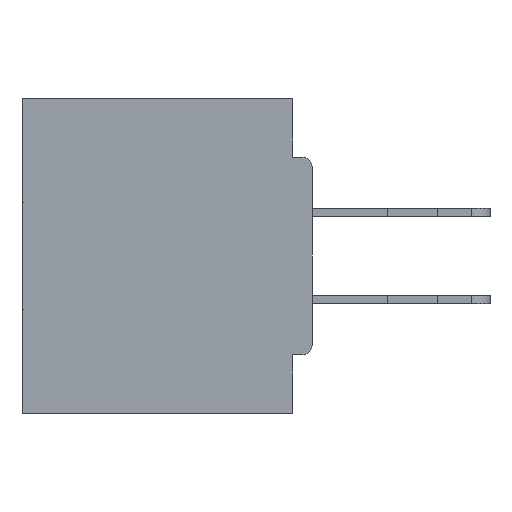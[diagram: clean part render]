
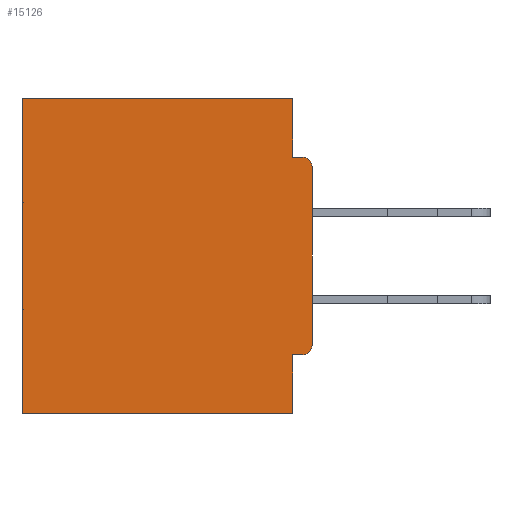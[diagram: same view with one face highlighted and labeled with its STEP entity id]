
A CAD part, left-side view. The second image highlights one B-rep face of the part: STEP entity #15126.
In plain terms, the highlighted planar face has unit normal (-1, 0, 0).
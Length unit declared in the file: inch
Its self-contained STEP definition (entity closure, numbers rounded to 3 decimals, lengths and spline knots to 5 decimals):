
#504 = LINE ( 'NONE', #10023, #5529 ) ;
#1073 = CARTESIAN_POINT ( 'NONE',  ( 0.298, 0.015, -0.4065 ) ) ;
#1632 = EDGE_LOOP ( 'NONE', ( #32074, #9726, #23702, #25996, #10552, #6517, #4201, #10667, #2565, #26177 ) ) ;
#1644 = EDGE_CURVE ( 'NONE', #39556, #12354, #32838, .T. ) ;
#1906 = CARTESIAN_POINT ( 'NONE',  ( 0.298, 0.031, -0.4065 ) ) ;
#2469 = FACE_OUTER_BOUND ( 'NONE', #1632, .T. ) ;
#2565 = ORIENTED_EDGE ( 'NONE', *, *, #34177, .T. ) ;
#2926 = LINE ( 'NONE', #29015, #8430 ) ;
#3971 = EDGE_CURVE ( 'NONE', #5080, #12354, #32629, .T. ) ;
#4201 = ORIENTED_EDGE ( 'NONE', *, *, #24103, .F. ) ;
#5080 = VERTEX_POINT ( 'NONE', #30779 ) ;
#5529 = VECTOR ( 'NONE', #22560, 39.37008 ) ;
#5671 = DIRECTION ( 'NONE',  ( 0., 0., -1. ) ) ;
#6390 = DIRECTION ( 'NONE',  ( 0., 0., -1. ) ) ;
#6517 = ORIENTED_EDGE ( 'NONE', *, *, #10736, .F. ) ;
#7818 = CARTESIAN_POINT ( 'NONE',  ( 0.298, 0., 0. ) ) ;
#8029 = EDGE_CURVE ( 'NONE', #39330, #17224, #26797, .T. ) ;
#8430 = VECTOR ( 'NONE', #19400, 39.37008 ) ;
#8627 = AXIS2_PLACEMENT_3D ( 'NONE', #16144, #38424, #19344 ) ;
#8800 = LINE ( 'NONE', #11497, #19780 ) ;
#9360 = CARTESIAN_POINT ( 'NONE',  ( 0.298, 0.015, -0.1085 ) ) ;
#9726 = ORIENTED_EDGE ( 'NONE', *, *, #1644, .F. ) ;
#10023 = CARTESIAN_POINT ( 'NONE',  ( 0.298, 0., 0. ) ) ;
#10038 = CIRCLE ( 'NONE', #8627, 0.015 ) ;
#10053 = VECTOR ( 'NONE', #5671, 39.37008 ) ;
#10339 = LINE ( 'NONE', #15567, #19294 ) ;
#10552 = ORIENTED_EDGE ( 'NONE', *, *, #19890, .T. ) ;
#10667 = ORIENTED_EDGE ( 'NONE', *, *, #20920, .F. ) ;
#10736 = EDGE_CURVE ( 'NONE', #15590, #25500, #8800, .T. ) ;
#11012 = LINE ( 'NONE', #41060, #10053 ) ;
#11497 = CARTESIAN_POINT ( 'NONE',  ( 0.298, 0., -0.5 ) ) ;
#12354 = VERTEX_POINT ( 'NONE', #16309 ) ;
#12624 = VERTEX_POINT ( 'NONE', #1073 ) ;
#13144 = DIRECTION ( 'NONE',  ( 0., -1., 0. ) ) ;
#13216 = VECTOR ( 'NONE', #37300, 39.37008 ) ;
#14861 = VECTOR ( 'NONE', #13144, 39.37008 ) ;
#15126 = ADVANCED_FACE ( 'NONE', ( #2469 ), #41079, .F. ) ;
#15567 = CARTESIAN_POINT ( 'NONE',  ( 0.298, 0., -0.4065 ) ) ;
#15590 = VERTEX_POINT ( 'NONE', #34446 ) ;
#15785 = CARTESIAN_POINT ( 'NONE',  ( 0.298, 0.031, 0. ) ) ;
#16144 = CARTESIAN_POINT ( 'NONE',  ( 0.298, 0.015, -0.3915 ) ) ;
#16309 = CARTESIAN_POINT ( 'NONE',  ( 0.298, 0.015, -0.0935 ) ) ;
#17224 = VERTEX_POINT ( 'NONE', #37334 ) ;
#18289 = VECTOR ( 'NONE', #39715, 39.37008 ) ;
#18800 = EDGE_CURVE ( 'NONE', #5080, #19635, #504, .T. ) ;
#18860 = CARTESIAN_POINT ( 'NONE',  ( 0.298, 0.46, -0.5 ) ) ;
#18916 = DIRECTION ( 'NONE',  ( 0., 1., 0. ) ) ;
#19294 = VECTOR ( 'NONE', #18916, 39.37008 ) ;
#19344 = DIRECTION ( 'NONE',  ( 0., 0., -1. ) ) ;
#19400 = DIRECTION ( 'NONE',  ( 0., 0., -1. ) ) ;
#19635 = VERTEX_POINT ( 'NONE', #39042 ) ;
#19780 = VECTOR ( 'NONE', #21122, 39.37008 ) ;
#19890 = EDGE_CURVE ( 'NONE', #17224, #25500, #2926, .T. ) ;
#20398 = CARTESIAN_POINT ( 'NONE',  ( 0.298, 0.031, -0.0935 ) ) ;
#20920 = EDGE_CURVE ( 'NONE', #12624, #30329, #10339, .T. ) ;
#21122 = DIRECTION ( 'NONE',  ( 0., 1., 0. ) ) ;
#22560 = DIRECTION ( 'NONE',  ( 0., 0., -1. ) ) ;
#23702 = ORIENTED_EDGE ( 'NONE', *, *, #26275, .F. ) ;
#24103 = EDGE_CURVE ( 'NONE', #30329, #15590, #30160, .T. ) ;
#25359 = DIRECTION ( 'NONE',  ( -1., 0., 0. ) ) ;
#25500 = VERTEX_POINT ( 'NONE', #18860 ) ;
#25996 = ORIENTED_EDGE ( 'NONE', *, *, #8029, .T. ) ;
#26177 = ORIENTED_EDGE ( 'NONE', *, *, #18800, .F. ) ;
#26275 = EDGE_CURVE ( 'NONE', #39330, #39556, #11012, .T. ) ;
#26797 = LINE ( 'NONE', #7818, #18289 ) ;
#28815 = DIRECTION ( 'NONE',  ( 1., 0., 0. ) ) ;
#29015 = CARTESIAN_POINT ( 'NONE',  ( 0.298, 0.46, 0. ) ) ;
#29329 = CARTESIAN_POINT ( 'NONE',  ( 0.298, 0., -0.0935 ) ) ;
#30160 = LINE ( 'NONE', #39994, #13216 ) ;
#30329 = VERTEX_POINT ( 'NONE', #1906 ) ;
#30779 = CARTESIAN_POINT ( 'NONE',  ( 0.298, 0., -0.1085 ) ) ;
#31103 = DIRECTION ( 'NONE',  ( 0., 0., -1. ) ) ;
#31507 = AXIS2_PLACEMENT_3D ( 'NONE', #34912, #28815, #6390 ) ;
#31741 = AXIS2_PLACEMENT_3D ( 'NONE', #9360, #25359, #31103 ) ;
#32074 = ORIENTED_EDGE ( 'NONE', *, *, #3971, .T. ) ;
#32629 = CIRCLE ( 'NONE', #31741, 0.015 ) ;
#32838 = LINE ( 'NONE', #29329, #14861 ) ;
#34177 = EDGE_CURVE ( 'NONE', #12624, #19635, #10038, .T. ) ;
#34446 = CARTESIAN_POINT ( 'NONE',  ( 0.298, 0.031, -0.5 ) ) ;
#34912 = CARTESIAN_POINT ( 'NONE',  ( 0.298, 0., 0. ) ) ;
#37300 = DIRECTION ( 'NONE',  ( 0., 0., -1. ) ) ;
#37334 = CARTESIAN_POINT ( 'NONE',  ( 0.298, 0.46, 0. ) ) ;
#38424 = DIRECTION ( 'NONE',  ( -1., 0., 0. ) ) ;
#39042 = CARTESIAN_POINT ( 'NONE',  ( 0.298, 0., -0.3915 ) ) ;
#39330 = VERTEX_POINT ( 'NONE', #15785 ) ;
#39556 = VERTEX_POINT ( 'NONE', #20398 ) ;
#39715 = DIRECTION ( 'NONE',  ( 0., 1., 0. ) ) ;
#39994 = CARTESIAN_POINT ( 'NONE',  ( 0.298, 0.031, -0.5 ) ) ;
#41060 = CARTESIAN_POINT ( 'NONE',  ( 0.298, 0.031, -0.5 ) ) ;
#41079 = PLANE ( 'NONE',  #31507 ) ;
